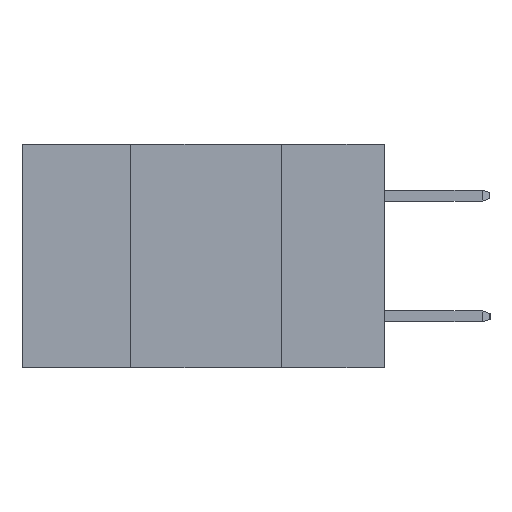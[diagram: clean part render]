
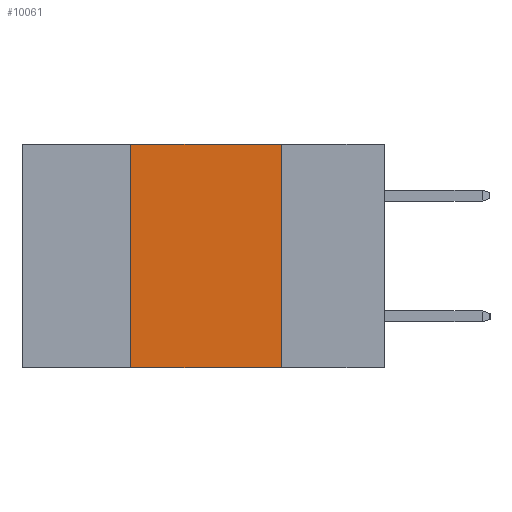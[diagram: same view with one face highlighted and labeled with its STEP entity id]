
A CAD part, left-side view. The second image highlights one B-rep face of the part: STEP entity #10061.
In plain terms, the highlighted planar face has unit normal (-1, 0, 0).
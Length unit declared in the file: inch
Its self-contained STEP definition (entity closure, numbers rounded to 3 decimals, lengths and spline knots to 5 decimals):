
#187 = ORIENTED_EDGE ( 'NONE', *, *, #3589, .F. ) ;
#1306 = EDGE_CURVE ( 'NONE', #10121, #12202, #9703, .T. ) ;
#2065 = VECTOR ( 'NONE', #3569, 39.37008 ) ;
#2342 = LINE ( 'NONE', #9925, #4254 ) ;
#2352 = CARTESIAN_POINT ( 'NONE',  ( 0., 0.42, -0.37 ) ) ;
#2358 = VERTEX_POINT ( 'NONE', #9977 ) ;
#2586 = EDGE_CURVE ( 'NONE', #6363, #12202, #8052, .T. ) ;
#2672 = EDGE_CURVE ( 'NONE', #2358, #10121, #2342, .T. ) ;
#2944 = VECTOR ( 'NONE', #11358, 39.37008 ) ;
#3569 = DIRECTION ( 'NONE',  ( 0., 0., -1. ) ) ;
#3589 = EDGE_CURVE ( 'NONE', #6363, #2358, #4232, .T. ) ;
#3939 = VECTOR ( 'NONE', #11785, 39.37008 ) ;
#4232 = LINE ( 'NONE', #10947, #3939 ) ;
#4254 = VECTOR ( 'NONE', #9826, 39.37008 ) ;
#5016 = DIRECTION ( 'NONE',  ( 1., 0., 0. ) ) ;
#5109 = CARTESIAN_POINT ( 'NONE',  ( 0., 0.17, 0. ) ) ;
#5762 = ORIENTED_EDGE ( 'NONE', *, *, #1306, .F. ) ;
#6363 = VERTEX_POINT ( 'NONE', #2352 ) ;
#6529 = CARTESIAN_POINT ( 'NONE',  ( 0., 0.17, -0.37 ) ) ;
#6873 = EDGE_LOOP ( 'NONE', ( #5762, #9494, #187, #11112 ) ) ;
#6925 = PLANE ( 'NONE',  #8609 ) ;
#8052 = LINE ( 'NONE', #11421, #2944 ) ;
#8609 = AXIS2_PLACEMENT_3D ( 'NONE', #8855, #5016, #11697 ) ;
#8855 = CARTESIAN_POINT ( 'NONE',  ( 0., 0.6, 0. ) ) ;
#9494 = ORIENTED_EDGE ( 'NONE', *, *, #2672, .F. ) ;
#9703 = LINE ( 'NONE', #6529, #2065 ) ;
#9826 = DIRECTION ( 'NONE',  ( 0., -1., 0. ) ) ;
#9925 = CARTESIAN_POINT ( 'NONE',  ( 0., 0.6, 0. ) ) ;
#9977 = CARTESIAN_POINT ( 'NONE',  ( 0., 0.42, 0. ) ) ;
#10061 = ADVANCED_FACE ( 'NONE', ( #10809 ), #6925, .F. ) ;
#10121 = VERTEX_POINT ( 'NONE', #5109 ) ;
#10809 = FACE_OUTER_BOUND ( 'NONE', #6873, .T. ) ;
#10947 = CARTESIAN_POINT ( 'NONE',  ( 0., 0.42, -0.37 ) ) ;
#11112 = ORIENTED_EDGE ( 'NONE', *, *, #2586, .T. ) ;
#11358 = DIRECTION ( 'NONE',  ( 0., -1., 0. ) ) ;
#11421 = CARTESIAN_POINT ( 'NONE',  ( 0., 0.6, -0.37 ) ) ;
#11697 = DIRECTION ( 'NONE',  ( 0., 0., -1. ) ) ;
#11785 = DIRECTION ( 'NONE',  ( 0., 0., 1. ) ) ;
#12170 = CARTESIAN_POINT ( 'NONE',  ( 0., 0.17, -0.37 ) ) ;
#12202 = VERTEX_POINT ( 'NONE', #12170 ) ;
